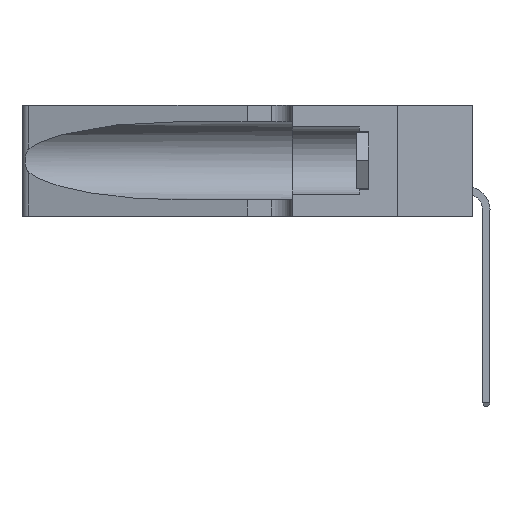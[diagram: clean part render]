
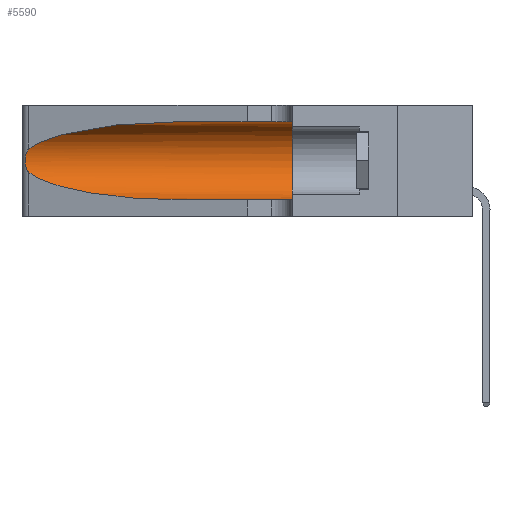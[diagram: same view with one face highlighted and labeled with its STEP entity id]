
A CAD part, left-side view. The second image highlights one B-rep face of the part: STEP entity #5590.
In plain terms, the highlighted cylindrical face has radius 3.308 mm (diameter 6.617 mm), a partial arc.
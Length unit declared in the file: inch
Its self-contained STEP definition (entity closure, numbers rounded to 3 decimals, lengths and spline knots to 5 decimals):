
#425 = CARTESIAN_POINT ( 'NONE',  ( 0.18966, 0.96281, 0.05475 ) ) ;
#631 = VECTOR ( 'NONE', #4224, 39.37008 ) ;
#1516 = VERTEX_POINT ( 'NONE', #30570 ) ;
#2187 = CARTESIAN_POINT ( 'NONE',  ( 0.18966, 0.96281, 0.31525 ) ) ;
#2274 = EDGE_CURVE ( 'NONE', #25115, #3886, #30660, .T. ) ;
#2289 = CARTESIAN_POINT ( 'NONE',  ( 0.25555, 1.22993, 0.14849 ) ) ;
#2655 = CARTESIAN_POINT ( 'NONE',  ( 0.25555, 1.22994, 0.2215 ) ) ;
#3886 = VERTEX_POINT ( 'NONE', #13671 ) ;
#4048 = AXIS2_PLACEMENT_3D ( 'NONE', #14064, #22570, #28105 ) ;
#4094 =( BOUNDED_CURVE ( )  B_SPLINE_CURVE ( 3, ( #11834, #6218, #425, #8858 ),
 .UNSPECIFIED., .F., .T. ) 
 B_SPLINE_CURVE_WITH_KNOTS ( ( 4, 4 ),
 ( 3.44316, 4.71239 ),
 .UNSPECIFIED. ) 
 CURVE ( )  GEOMETRIC_REPRESENTATION_ITEM ( )  RATIONAL_B_SPLINE_CURVE ( ( 1., 0.87, 0.87, 1. ) ) 
 REPRESENTATION_ITEM ( '' )  );
#4124 = EDGE_CURVE ( 'NONE', #3886, #20268, #4094, .T. ) ;
#4224 = DIRECTION ( 'NONE',  ( 0., -1., 0. ) ) ;
#5590 = ADVANCED_FACE ( 'NONE', ( #24483 ), #10183, .F. ) ;
#5638 = EDGE_LOOP ( 'NONE', ( #35960, #15905, #17755, #14793, #17462, #34568 ) ) ;
#6184 = EDGE_CURVE ( 'NONE', #11609, #35919, #11845, .T. ) ;
#6218 = CARTESIAN_POINT ( 'NONE',  ( 0.2373, 1.15595, 0.08982 ) ) ;
#7069 = EDGE_CURVE ( 'NONE', #1516, #25115, #34488, .T. ) ;
#7920 = CARTESIAN_POINT ( 'NONE',  ( 0.25487, 1.22718, 0.22369 ) ) ;
#8164 = CARTESIAN_POINT ( 'NONE',  ( 0.26075, 1.23896, 0.178 ) ) ;
#8288 = DIRECTION ( 'NONE',  ( 0., 0., 1. ) ) ;
#8858 = CARTESIAN_POINT ( 'NONE',  ( 0.1305, 0.72297, 0.05475 ) ) ;
#10183 = CYLINDRICAL_SURFACE ( 'NONE', #4048, 0.13025 ) ;
#10776 = CARTESIAN_POINT ( 'NONE',  ( 0.25787, 1.23484, 0.2124 ) ) ;
#11018 = CARTESIAN_POINT ( 'NONE',  ( 0.25487, 1.22718, 0.14631 ) ) ;
#11609 = VERTEX_POINT ( 'NONE', #35092 ) ;
#11834 = CARTESIAN_POINT ( 'NONE',  ( 0.25487, 1.22718, 0.14631 ) ) ;
#11845 = CIRCLE ( 'NONE', #33493, 0.13025 ) ;
#11964 = EDGE_CURVE ( 'NONE', #1516, #11609, #22545, .T. ) ;
#13659 = CARTESIAN_POINT ( 'NONE',  ( 0.25856, 1.23593, 0.16098 ) ) ;
#13671 = CARTESIAN_POINT ( 'NONE',  ( 0.25487, 1.22718, 0.14631 ) ) ;
#13807 = CARTESIAN_POINT ( 'NONE',  ( 0.2373, 1.15595, 0.28018 ) ) ;
#14064 = CARTESIAN_POINT ( 'NONE',  ( 0.1305, 1.61858, 0.185 ) ) ;
#14793 = ORIENTED_EDGE ( 'NONE', *, *, #19518, .T. ) ;
#14913 = VECTOR ( 'NONE', #35682, 39.37008 ) ;
#15787 = CARTESIAN_POINT ( 'NONE',  ( 0.1305, 1.61858, 0.31525 ) ) ;
#15905 = ORIENTED_EDGE ( 'NONE', *, *, #2274, .T. ) ;
#15938 = CARTESIAN_POINT ( 'NONE',  ( 0.25487, 1.22718, 0.22369 ) ) ;
#16696 = CARTESIAN_POINT ( 'NONE',  ( 0.26017, 1.23833, 0.17102 ) ) ;
#16937 = CARTESIAN_POINT ( 'NONE',  ( 0.1305, 0.72297, 0.05475 ) ) ;
#17462 = ORIENTED_EDGE ( 'NONE', *, *, #6184, .F. ) ;
#17755 = ORIENTED_EDGE ( 'NONE', *, *, #4124, .T. ) ;
#18111 = CARTESIAN_POINT ( 'NONE',  ( 0.1305, 1.61858, 0.05475 ) ) ;
#19353 = CARTESIAN_POINT ( 'NONE',  ( 0.1305, 0.72297, 0.31525 ) ) ;
#19461 = CARTESIAN_POINT ( 'NONE',  ( 0.25639, 1.23186, 0.15144 ) ) ;
#19518 = EDGE_CURVE ( 'NONE', #20268, #35919, #31095, .T. ) ;
#19691 = DIRECTION ( 'NONE',  ( 0., 1., 0. ) ) ;
#20268 = VERTEX_POINT ( 'NONE', #16937 ) ;
#21498 = CARTESIAN_POINT ( 'NONE',  ( 0.1305, 0.35, 0.185 ) ) ;
#22545 = LINE ( 'NONE', #15787, #14913 ) ;
#22570 = DIRECTION ( 'NONE',  ( 0., -1., 0. ) ) ;
#22652 = CARTESIAN_POINT ( 'NONE',  ( 0.26018, 1.23835, 0.19895 ) ) ;
#24483 = FACE_OUTER_BOUND ( 'NONE', #5638, .T. ) ;
#25058 = CARTESIAN_POINT ( 'NONE',  ( 0.25487, 1.22718, 0.22369 ) ) ;
#25115 = VERTEX_POINT ( 'NONE', #15938 ) ;
#28105 = DIRECTION ( 'NONE',  ( 0., 0., -1. ) ) ;
#30570 = CARTESIAN_POINT ( 'NONE',  ( 0.1305, 0.72297, 0.31525 ) ) ;
#30660 = B_SPLINE_CURVE_WITH_KNOTS ( 'NONE', 3,
 ( #7920, #2655, #31136, #10776, #30772, #22652, #33889, #8164, #16696, #13659, #36464, #19461, #2289, #11018 ),
 .UNSPECIFIED., .F., .F.,
 ( 4, 2, 2, 2, 2, 2, 4 ),
 ( 0., 0.00027, 0.00053, 0.00107, 0.0016, 0.00187, 0.00214 ),
 .UNSPECIFIED. ) ;
#30772 = CARTESIAN_POINT ( 'NONE',  ( 0.25854, 1.2359, 0.20912 ) ) ;
#31095 = LINE ( 'NONE', #18111, #631 ) ;
#31136 = CARTESIAN_POINT ( 'NONE',  ( 0.25639, 1.23184, 0.21858 ) ) ;
#33493 = AXIS2_PLACEMENT_3D ( 'NONE', #21498, #19691, #8288 ) ;
#33889 = CARTESIAN_POINT ( 'NONE',  ( 0.26075, 1.23896, 0.19203 ) ) ;
#34488 =( BOUNDED_CURVE ( )  B_SPLINE_CURVE ( 3, ( #19353, #2187, #13807, #25058 ),
 .UNSPECIFIED., .F., .T. ) 
 B_SPLINE_CURVE_WITH_KNOTS ( ( 4, 4 ),
 ( 1.5708, 2.84003 ),
 .UNSPECIFIED. ) 
 CURVE ( )  GEOMETRIC_REPRESENTATION_ITEM ( )  RATIONAL_B_SPLINE_CURVE ( ( 1., 0.87, 0.87, 1. ) ) 
 REPRESENTATION_ITEM ( '' )  );
#34568 = ORIENTED_EDGE ( 'NONE', *, *, #11964, .F. ) ;
#35092 = CARTESIAN_POINT ( 'NONE',  ( 0.1305, 0.35, 0.31525 ) ) ;
#35682 = DIRECTION ( 'NONE',  ( 0., -1., 0. ) ) ;
#35919 = VERTEX_POINT ( 'NONE', #36857 ) ;
#35960 = ORIENTED_EDGE ( 'NONE', *, *, #7069, .T. ) ;
#36464 = CARTESIAN_POINT ( 'NONE',  ( 0.25789, 1.23486, 0.15765 ) ) ;
#36857 = CARTESIAN_POINT ( 'NONE',  ( 0.1305, 0.35, 0.05475 ) ) ;
